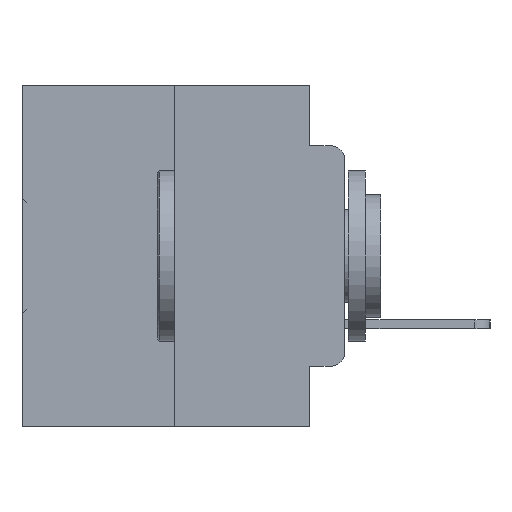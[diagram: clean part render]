
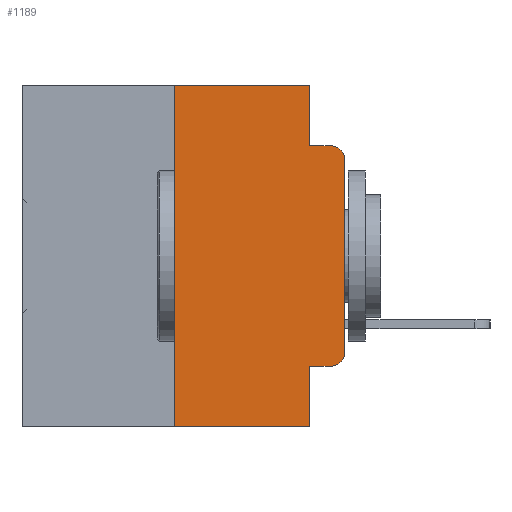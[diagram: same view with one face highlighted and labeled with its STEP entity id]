
A CAD part, left-side view. The second image highlights one B-rep face of the part: STEP entity #1189.
In plain terms, the highlighted planar face has unit normal (-1, 0, 0).
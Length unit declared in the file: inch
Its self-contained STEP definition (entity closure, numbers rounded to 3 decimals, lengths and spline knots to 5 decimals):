
#1189 = ADVANCED_FACE ( 'NONE', ( #19432 ), #7130, .F. ) ;
#1285 = ORIENTED_EDGE ( 'NONE', *, *, #25043, .T. ) ;
#1414 = DIRECTION ( 'NONE',  ( 0., 0., 1. ) ) ;
#1522 = DIRECTION ( 'NONE',  ( 0., -1., 0. ) ) ;
#1948 = EDGE_CURVE ( 'NONE', #7351, #2141, #31554, .T. ) ;
#2077 = CARTESIAN_POINT ( 'NONE',  ( 0., 0., -0.3915 ) ) ;
#2124 = ORIENTED_EDGE ( 'NONE', *, *, #23303, .F. ) ;
#2129 = VECTOR ( 'NONE', #27298, 39.37008 ) ;
#2141 = VERTEX_POINT ( 'NONE', #21824 ) ;
#2703 = LINE ( 'NONE', #23448, #21657 ) ;
#2716 = CARTESIAN_POINT ( 'NONE',  ( 0., 0., 0. ) ) ;
#2836 = LINE ( 'NONE', #16012, #11333 ) ;
#3251 = CARTESIAN_POINT ( 'NONE',  ( 0., 0.25, 0. ) ) ;
#3730 = VERTEX_POINT ( 'NONE', #14302 ) ;
#4015 = LINE ( 'NONE', #17009, #16925 ) ;
#4347 = EDGE_LOOP ( 'NONE', ( #32840, #1285, #2124, #9007, #16669, #30132, #31681, #20716, #22304, #9423 ) ) ;
#4826 = DIRECTION ( 'NONE',  ( 1., 0., 0. ) ) ;
#4986 = CARTESIAN_POINT ( 'NONE',  ( 0., 0.02, -0.4115 ) ) ;
#5819 = CIRCLE ( 'NONE', #26712, 0.02 ) ;
#6068 = CARTESIAN_POINT ( 'NONE',  ( 0., 0.051, -0.0885 ) ) ;
#6092 = EDGE_CURVE ( 'NONE', #3730, #17733, #29352, .T. ) ;
#6298 = AXIS2_PLACEMENT_3D ( 'NONE', #25158, #9770, #27660 ) ;
#6924 = VECTOR ( 'NONE', #17954, 39.37008 ) ;
#7130 = PLANE ( 'NONE',  #17685 ) ;
#7351 = VERTEX_POINT ( 'NONE', #2077 ) ;
#8609 = VERTEX_POINT ( 'NONE', #18275 ) ;
#9006 = VERTEX_POINT ( 'NONE', #32441 ) ;
#9007 = ORIENTED_EDGE ( 'NONE', *, *, #14704, .F. ) ;
#9258 = DIRECTION ( 'NONE',  ( 0., 0., -1. ) ) ;
#9423 = ORIENTED_EDGE ( 'NONE', *, *, #23948, .T. ) ;
#9770 = DIRECTION ( 'NONE',  ( -1., 0., 0. ) ) ;
#10186 = CARTESIAN_POINT ( 'NONE',  ( 0., 0.473, 0. ) ) ;
#11333 = VECTOR ( 'NONE', #18741, 39.37008 ) ;
#11433 = LINE ( 'NONE', #19406, #30915 ) ;
#11610 = CARTESIAN_POINT ( 'NONE',  ( 0., 0.02, -0.1085 ) ) ;
#12336 = CIRCLE ( 'NONE', #6298, 0.02 ) ;
#12969 = EDGE_CURVE ( 'NONE', #8609, #17124, #11433, .T. ) ;
#13221 = DIRECTION ( 'NONE',  ( 0., -1., 0. ) ) ;
#14170 = DIRECTION ( 'NONE',  ( 0., 0., -1. ) ) ;
#14302 = CARTESIAN_POINT ( 'NONE',  ( 0., 0.051, -0.4115 ) ) ;
#14321 = EDGE_CURVE ( 'NONE', #8609, #17733, #2836, .T. ) ;
#14547 = LINE ( 'NONE', #23068, #6924 ) ;
#14704 = EDGE_CURVE ( 'NONE', #23621, #27933, #19805, .T. ) ;
#16012 = CARTESIAN_POINT ( 'NONE',  ( 0., 0.473, -0.5 ) ) ;
#16669 = ORIENTED_EDGE ( 'NONE', *, *, #22561, .F. ) ;
#16925 = VECTOR ( 'NONE', #1522, 39.37008 ) ;
#17009 = CARTESIAN_POINT ( 'NONE',  ( 0., 0.051, -0.0885 ) ) ;
#17124 = VERTEX_POINT ( 'NONE', #3251 ) ;
#17685 = AXIS2_PLACEMENT_3D ( 'NONE', #10186, #4826, #9258 ) ;
#17733 = VERTEX_POINT ( 'NONE', #31107 ) ;
#17954 = DIRECTION ( 'NONE',  ( 0., -1., 0. ) ) ;
#18275 = CARTESIAN_POINT ( 'NONE',  ( 0., 0.25, -0.5 ) ) ;
#18352 = CARTESIAN_POINT ( 'NONE',  ( 0., 0.051, 0. ) ) ;
#18741 = DIRECTION ( 'NONE',  ( 0., -1., 0. ) ) ;
#18990 = VECTOR ( 'NONE', #30305, 39.37008 ) ;
#19406 = CARTESIAN_POINT ( 'NONE',  ( 0., 0.25, 0. ) ) ;
#19432 = FACE_OUTER_BOUND ( 'NONE', #4347, .T. ) ;
#19805 = LINE ( 'NONE', #27806, #18990 ) ;
#20641 = VERTEX_POINT ( 'NONE', #4986 ) ;
#20716 = ORIENTED_EDGE ( 'NONE', *, *, #6092, .F. ) ;
#21657 = VECTOR ( 'NONE', #13221, 39.37008 ) ;
#21824 = CARTESIAN_POINT ( 'NONE',  ( 0., 0., -0.1085 ) ) ;
#22304 = ORIENTED_EDGE ( 'NONE', *, *, #32302, .T. ) ;
#22561 = EDGE_CURVE ( 'NONE', #17124, #23621, #14547, .T. ) ;
#23068 = CARTESIAN_POINT ( 'NONE',  ( 0., 0.473, 0. ) ) ;
#23303 = EDGE_CURVE ( 'NONE', #27933, #9006, #4015, .T. ) ;
#23332 = VECTOR ( 'NONE', #32942, 39.37008 ) ;
#23448 = CARTESIAN_POINT ( 'NONE',  ( 0., 0.051, -0.4115 ) ) ;
#23621 = VERTEX_POINT ( 'NONE', #18352 ) ;
#23948 = EDGE_CURVE ( 'NONE', #20641, #7351, #12336, .T. ) ;
#24798 = CARTESIAN_POINT ( 'NONE',  ( 0., 0.051, 0. ) ) ;
#25043 = EDGE_CURVE ( 'NONE', #2141, #9006, #5819, .T. ) ;
#25158 = CARTESIAN_POINT ( 'NONE',  ( 0., 0.02, -0.3915 ) ) ;
#26712 = AXIS2_PLACEMENT_3D ( 'NONE', #11610, #29410, #14170 ) ;
#27298 = DIRECTION ( 'NONE',  ( 0., 0., -1. ) ) ;
#27660 = DIRECTION ( 'NONE',  ( 0., 0., -1. ) ) ;
#27806 = CARTESIAN_POINT ( 'NONE',  ( 0., 0.051, 0. ) ) ;
#27933 = VERTEX_POINT ( 'NONE', #6068 ) ;
#29352 = LINE ( 'NONE', #24798, #2129 ) ;
#29410 = DIRECTION ( 'NONE',  ( -1., 0., 0. ) ) ;
#30132 = ORIENTED_EDGE ( 'NONE', *, *, #12969, .F. ) ;
#30305 = DIRECTION ( 'NONE',  ( 0., 0., -1. ) ) ;
#30915 = VECTOR ( 'NONE', #1414, 39.37008 ) ;
#31107 = CARTESIAN_POINT ( 'NONE',  ( 0., 0.051, -0.5 ) ) ;
#31554 = LINE ( 'NONE', #2716, #23332 ) ;
#31681 = ORIENTED_EDGE ( 'NONE', *, *, #14321, .T. ) ;
#32302 = EDGE_CURVE ( 'NONE', #3730, #20641, #2703, .T. ) ;
#32441 = CARTESIAN_POINT ( 'NONE',  ( 0., 0.02, -0.0885 ) ) ;
#32840 = ORIENTED_EDGE ( 'NONE', *, *, #1948, .T. ) ;
#32942 = DIRECTION ( 'NONE',  ( 0., 0., 1. ) ) ;
